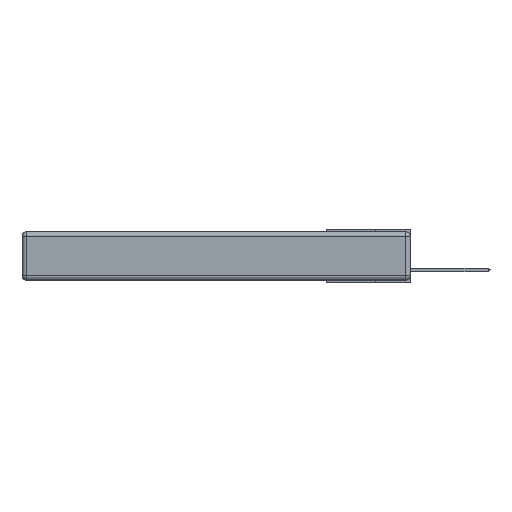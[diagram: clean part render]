
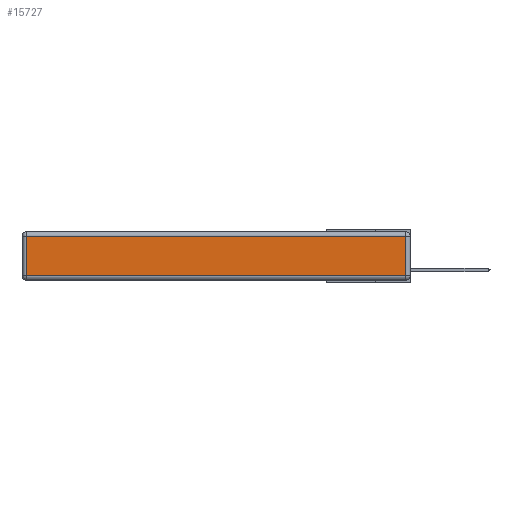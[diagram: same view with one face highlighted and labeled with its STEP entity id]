
A CAD part, left-side view. The second image highlights one B-rep face of the part: STEP entity #15727.
In plain terms, the highlighted planar face has unit normal (-1, 0, 0).
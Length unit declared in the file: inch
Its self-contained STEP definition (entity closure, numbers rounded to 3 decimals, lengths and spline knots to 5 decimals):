
#93 = VERTEX_POINT ( 'NONE', #14575 ) ;
#306 = VECTOR ( 'NONE', #2818, 39.37008 ) ;
#1382 = CARTESIAN_POINT ( 'NONE',  ( 0., 0., -0.313 ) ) ;
#1559 = AXIS2_PLACEMENT_3D ( 'NONE', #23150, #5170, #11317 ) ;
#2064 = LINE ( 'NONE', #16289, #17142 ) ;
#2412 = LINE ( 'NONE', #18382, #15589 ) ;
#2425 = EDGE_CURVE ( 'NONE', #93, #24522, #2412, .T. ) ;
#2818 = DIRECTION ( 'NONE',  ( 0., 1., 0. ) ) ;
#3533 = CARTESIAN_POINT ( 'NONE',  ( 0., 2.72, -0.313 ) ) ;
#3611 = ORIENTED_EDGE ( 'NONE', *, *, #13934, .T. ) ;
#5170 = DIRECTION ( 'NONE',  ( -1., 0., 0. ) ) ;
#5415 = DIRECTION ( 'NONE',  ( 0., -1., 0. ) ) ;
#6362 = DIRECTION ( 'NONE',  ( 0., 0., -1. ) ) ;
#6574 = LINE ( 'NONE', #15179, #306 ) ;
#6627 = CARTESIAN_POINT ( 'NONE',  ( 0., 0.03, -0.313 ) ) ;
#6812 = FACE_OUTER_BOUND ( 'NONE', #16149, .T. ) ;
#8483 = LINE ( 'NONE', #1382, #18510 ) ;
#11317 = DIRECTION ( 'NONE',  ( 0., 0., 1. ) ) ;
#11827 = ORIENTED_EDGE ( 'NONE', *, *, #20434, .T. ) ;
#13934 = EDGE_CURVE ( 'NONE', #17191, #22729, #2064, .T. ) ;
#14575 = CARTESIAN_POINT ( 'NONE',  ( 0., 2.72, -0.03 ) ) ;
#15179 = CARTESIAN_POINT ( 'NONE',  ( 0., 2.75, -0.03 ) ) ;
#15589 = VECTOR ( 'NONE', #6362, 39.37008 ) ;
#15727 = ADVANCED_FACE ( 'NONE', ( #6812 ), #23321, .T. ) ;
#16149 = EDGE_LOOP ( 'NONE', ( #20919, #3611, #11827, #18217 ) ) ;
#16289 = CARTESIAN_POINT ( 'NONE',  ( 0., 0.03, -0.343 ) ) ;
#17142 = VECTOR ( 'NONE', #22223, 39.37008 ) ;
#17191 = VERTEX_POINT ( 'NONE', #6627 ) ;
#18217 = ORIENTED_EDGE ( 'NONE', *, *, #2425, .T. ) ;
#18382 = CARTESIAN_POINT ( 'NONE',  ( 0., 2.72, -0.343 ) ) ;
#18510 = VECTOR ( 'NONE', #5415, 39.37008 ) ;
#20434 = EDGE_CURVE ( 'NONE', #22729, #93, #6574, .T. ) ;
#20462 = EDGE_CURVE ( 'NONE', #24522, #17191, #8483, .T. ) ;
#20919 = ORIENTED_EDGE ( 'NONE', *, *, #20462, .T. ) ;
#22223 = DIRECTION ( 'NONE',  ( 0., 0., 1. ) ) ;
#22729 = VERTEX_POINT ( 'NONE', #25766 ) ;
#23150 = CARTESIAN_POINT ( 'NONE',  ( 0., 0., -0.343 ) ) ;
#23321 = PLANE ( 'NONE',  #1559 ) ;
#24522 = VERTEX_POINT ( 'NONE', #3533 ) ;
#25766 = CARTESIAN_POINT ( 'NONE',  ( 0., 0.03, -0.03 ) ) ;
